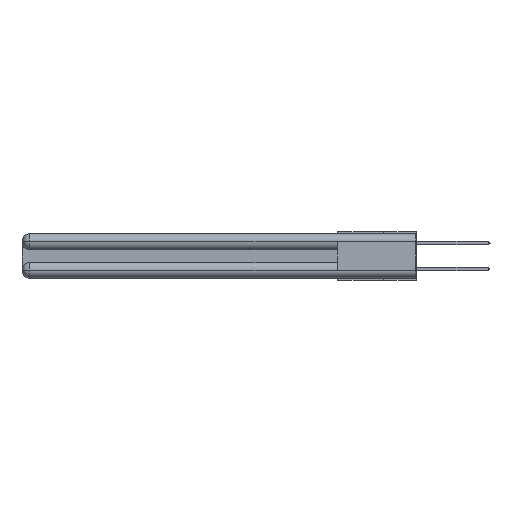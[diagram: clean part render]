
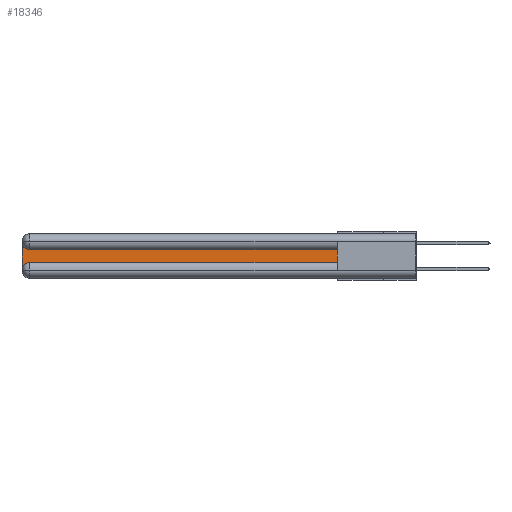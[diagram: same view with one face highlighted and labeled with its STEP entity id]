
A CAD part, left-side view. The second image highlights one B-rep face of the part: STEP entity #18346.
In plain terms, the highlighted planar face has unit normal (-1, 0, 0).
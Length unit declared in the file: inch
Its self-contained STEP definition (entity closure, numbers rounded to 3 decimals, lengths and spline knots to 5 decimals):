
#982 = DIRECTION ( 'NONE',  ( 0., 0., -1. ) ) ;
#2043 = CARTESIAN_POINT ( 'NONE',  ( 0.075, 2.94, -0.1225 ) ) ;
#2547 = VERTEX_POINT ( 'NONE', #26059 ) ;
#2633 = CIRCLE ( 'NONE', #15620, 0.06 ) ;
#2975 = DIRECTION ( 'NONE',  ( 1., 0., 0. ) ) ;
#3352 = CARTESIAN_POINT ( 'NONE',  ( 0.075, 0.6, -0.2175 ) ) ;
#3884 = ORIENTED_EDGE ( 'NONE', *, *, #34085, .T. ) ;
#4307 = ORIENTED_EDGE ( 'NONE', *, *, #18913, .T. ) ;
#4329 = LINE ( 'NONE', #3352, #11857 ) ;
#5512 = LINE ( 'NONE', #11976, #29319 ) ;
#5527 = DIRECTION ( 'NONE',  ( 0., 0., -1. ) ) ;
#5881 = CARTESIAN_POINT ( 'NONE',  ( 0.075, 2.94, -0.0625 ) ) ;
#6356 = LINE ( 'NONE', #11988, #26042 ) ;
#6565 = ORIENTED_EDGE ( 'NONE', *, *, #28015, .T. ) ;
#6872 = VERTEX_POINT ( 'NONE', #18750 ) ;
#8142 = FACE_OUTER_BOUND ( 'NONE', #16036, .T. ) ;
#8736 = VECTOR ( 'NONE', #25464, 39.37008 ) ;
#9166 = DIRECTION ( 'NONE',  ( 0., -1., 0. ) ) ;
#9560 = CARTESIAN_POINT ( 'NONE',  ( 0.075, 2.94, -0.2175 ) ) ;
#10917 = DIRECTION ( 'NONE',  ( 0., 0., -1. ) ) ;
#11211 = DIRECTION ( 'NONE',  ( 0., 0., 1. ) ) ;
#11241 = VERTEX_POINT ( 'NONE', #2043 ) ;
#11857 = VECTOR ( 'NONE', #11211, 39.37008 ) ;
#11976 = CARTESIAN_POINT ( 'NONE',  ( 0.075, 0.6, -0.2175 ) ) ;
#11988 = CARTESIAN_POINT ( 'NONE',  ( 0.075, 0.6, -0.1225 ) ) ;
#11993 = CARTESIAN_POINT ( 'NONE',  ( 0.075, 3., -0.2175 ) ) ;
#13076 = CARTESIAN_POINT ( 'NONE',  ( 0.075, 0.6, -0.2175 ) ) ;
#13542 = CARTESIAN_POINT ( 'NONE',  ( 0.075, 3., -0.1225 ) ) ;
#13726 = DIRECTION ( 'NONE',  ( 1., 0., 0. ) ) ;
#14000 = EDGE_CURVE ( 'NONE', #31115, #19390, #5512, .T. ) ;
#14393 = EDGE_CURVE ( 'NONE', #2547, #31115, #15938, .T. ) ;
#15620 = AXIS2_PLACEMENT_3D ( 'NONE', #5881, #19324, #10917 ) ;
#15668 = EDGE_CURVE ( 'NONE', #6872, #2547, #16683, .T. ) ;
#15938 = CIRCLE ( 'NONE', #22029, 0.06 ) ;
#16036 = EDGE_LOOP ( 'NONE', ( #6565, #4307, #17584, #22172, #18931, #3884 ) ) ;
#16683 = LINE ( 'NONE', #11993, #8736 ) ;
#17584 = ORIENTED_EDGE ( 'NONE', *, *, #15668, .T. ) ;
#18346 = ADVANCED_FACE ( 'NONE', ( #8142 ), #24426, .F. ) ;
#18750 = CARTESIAN_POINT ( 'NONE',  ( 0.075, 3., -0.0625 ) ) ;
#18913 = EDGE_CURVE ( 'NONE', #11241, #6872, #2633, .T. ) ;
#18931 = ORIENTED_EDGE ( 'NONE', *, *, #14000, .T. ) ;
#19324 = DIRECTION ( 'NONE',  ( 1., 0., 0. ) ) ;
#19390 = VERTEX_POINT ( 'NONE', #13076 ) ;
#22029 = AXIS2_PLACEMENT_3D ( 'NONE', #29673, #13726, #5527 ) ;
#22172 = ORIENTED_EDGE ( 'NONE', *, *, #14393, .T. ) ;
#22963 = CARTESIAN_POINT ( 'NONE',  ( 0.075, 0.6, -0.1225 ) ) ;
#24426 = PLANE ( 'NONE',  #29444 ) ;
#25464 = DIRECTION ( 'NONE',  ( 0., 0., -1. ) ) ;
#26042 = VECTOR ( 'NONE', #30652, 39.37008 ) ;
#26059 = CARTESIAN_POINT ( 'NONE',  ( 0.075, 3., -0.2775 ) ) ;
#27202 = VERTEX_POINT ( 'NONE', #22963 ) ;
#28015 = EDGE_CURVE ( 'NONE', #27202, #11241, #6356, .T. ) ;
#29319 = VECTOR ( 'NONE', #9166, 39.37008 ) ;
#29444 = AXIS2_PLACEMENT_3D ( 'NONE', #13542, #2975, #982 ) ;
#29673 = CARTESIAN_POINT ( 'NONE',  ( 0.075, 2.94, -0.2775 ) ) ;
#30652 = DIRECTION ( 'NONE',  ( 0., 1., 0. ) ) ;
#31115 = VERTEX_POINT ( 'NONE', #9560 ) ;
#34085 = EDGE_CURVE ( 'NONE', #19390, #27202, #4329, .T. ) ;
